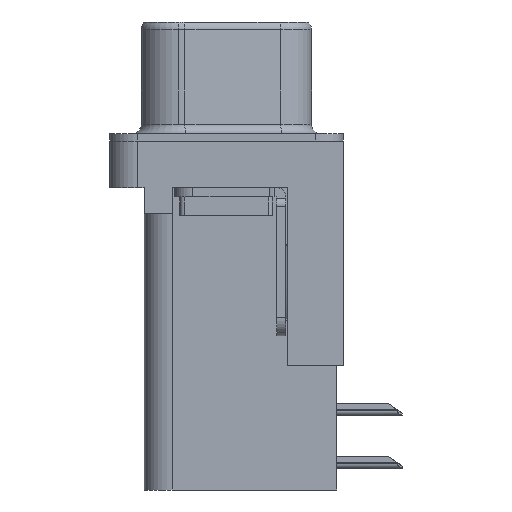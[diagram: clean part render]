
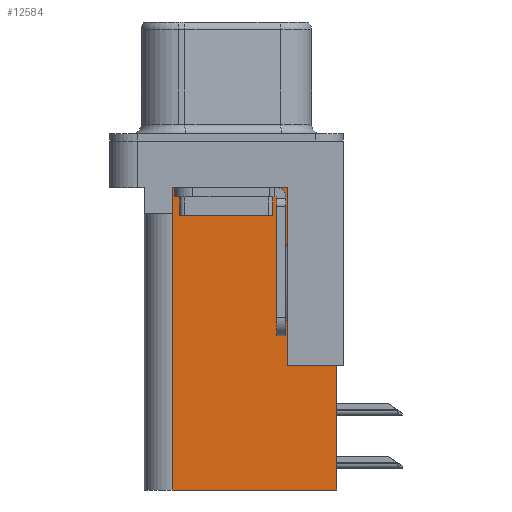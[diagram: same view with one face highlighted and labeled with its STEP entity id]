
A CAD part, left-side view. The second image highlights one B-rep face of the part: STEP entity #12584.
In plain terms, the highlighted planar face has unit normal (-1, 0, 0).
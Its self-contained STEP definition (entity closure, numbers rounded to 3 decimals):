
#171 = CARTESIAN_POINT ( 'NONE',  ( 3.7, -3.295, -18.76 ) ) ;
#661 = CARTESIAN_POINT ( 'NONE',  ( 3.7, 2.895, -3.9 ) ) ;
#1415 = CARTESIAN_POINT ( 'NONE',  ( 3.7, -3.295, -18.76 ) ) ;
#1554 = VECTOR ( 'NONE', #4974, 1000. ) ;
#1635 = LINE ( 'NONE', #19771, #1554 ) ;
#2069 = CARTESIAN_POINT ( 'NONE',  ( 3.7, -3.295, -2.5 ) ) ;
#3405 = VERTEX_POINT ( 'NONE', #21352 ) ;
#3714 = CARTESIAN_POINT ( 'NONE',  ( 3.7, 2.925, -18.76 ) ) ;
#3831 = CARTESIAN_POINT ( 'NONE',  ( 3.7, -6.295, -12.05 ) ) ;
#3982 = EDGE_LOOP ( 'NONE', ( #12504, #12738, #13119, #13442, #16560, #17139, #17426, #17558 ) ) ;
#4039 = VERTEX_POINT ( 'NONE', #17982 ) ;
#4243 = DIRECTION ( 'NONE',  ( 0., 1., 0. ) ) ;
#4322 = CARTESIAN_POINT ( 'NONE',  ( 3.7, 2.895, -3.9 ) ) ;
#4974 = DIRECTION ( 'NONE',  ( 0., 1., 0. ) ) ;
#6095 = DIRECTION ( 'NONE',  ( 0., 1., 0. ) ) ;
#6292 = DIRECTION ( 'NONE',  ( 0., 0., 1. ) ) ;
#6376 = VECTOR ( 'NONE', #6292, 1000. ) ;
#6480 = VERTEX_POINT ( 'NONE', #16243 ) ;
#6636 = LINE ( 'NONE', #171, #6376 ) ;
#6810 = CARTESIAN_POINT ( 'NONE',  ( 3.7, 2.925, -3.9 ) ) ;
#6896 = EDGE_CURVE ( 'NONE', #7898, #15439, #16103, .T. ) ;
#6897 = VECTOR ( 'NONE', #17127, 1000. ) ;
#6919 = LINE ( 'NONE', #3831, #6897 ) ;
#7898 = VERTEX_POINT ( 'NONE', #18029 ) ;
#8158 = LINE ( 'NONE', #13703, #8191 ) ;
#8191 = VECTOR ( 'NONE', #13785, 1000. ) ;
#8558 = VECTOR ( 'NONE', #12336, 1000. ) ;
#8704 = LINE ( 'NONE', #14214, #8558 ) ;
#8971 = EDGE_CURVE ( 'NONE', #4039, #7898, #8704, .T. ) ;
#9115 = EDGE_CURVE ( 'NONE', #13469, #4039, #8158, .T. ) ;
#9572 = EDGE_CURVE ( 'NONE', #13469, #16283, #6919, .T. ) ;
#9633 = DIRECTION ( 'NONE',  ( 0., 0., 1. ) ) ;
#9721 = EDGE_CURVE ( 'NONE', #16283, #3405, #6636, .T. ) ;
#11568 = VECTOR ( 'NONE', #19275, 1000. ) ;
#11760 = LINE ( 'NONE', #4322, #11568 ) ;
#12336 = DIRECTION ( 'NONE',  ( 0., 1., 0. ) ) ;
#12504 = ORIENTED_EDGE ( 'NONE', *, *, #18961, .T. ) ;
#12584 = ADVANCED_FACE ( 'NONE', ( #23570 ), #13771, .F. ) ;
#12738 = ORIENTED_EDGE ( 'NONE', *, *, #21416, .T. ) ;
#13119 = ORIENTED_EDGE ( 'NONE', *, *, #23737, .T. ) ;
#13442 = ORIENTED_EDGE ( 'NONE', *, *, #6896, .F. ) ;
#13469 = VERTEX_POINT ( 'NONE', #21233 ) ;
#13703 = CARTESIAN_POINT ( 'NONE',  ( 3.7, -5.925, -2. ) ) ;
#13771 = PLANE ( 'NONE',  #21087 ) ;
#13785 = DIRECTION ( 'NONE',  ( 0., 0., -1. ) ) ;
#14214 = CARTESIAN_POINT ( 'NONE',  ( 3.7, -3.295, -18.76 ) ) ;
#14871 = CARTESIAN_POINT ( 'NONE',  ( 3.7, -3.295, -12.05 ) ) ;
#15439 = VERTEX_POINT ( 'NONE', #6810 ) ;
#15578 = DIRECTION ( 'NONE',  ( 1., 0., 0. ) ) ;
#16079 = VECTOR ( 'NONE', #9633, 1000. ) ;
#16103 = LINE ( 'NONE', #3714, #16079 ) ;
#16243 = CARTESIAN_POINT ( 'NONE',  ( 3.7, 2.895, -2.5 ) ) ;
#16283 = VERTEX_POINT ( 'NONE', #14871 ) ;
#16560 = ORIENTED_EDGE ( 'NONE', *, *, #8971, .F. ) ;
#17127 = DIRECTION ( 'NONE',  ( 0., 1., 0. ) ) ;
#17139 = ORIENTED_EDGE ( 'NONE', *, *, #9115, .F. ) ;
#17338 = VECTOR ( 'NONE', #6095, 1000. ) ;
#17344 = LINE ( 'NONE', #2069, #17338 ) ;
#17426 = ORIENTED_EDGE ( 'NONE', *, *, #9572, .T. ) ;
#17558 = ORIENTED_EDGE ( 'NONE', *, *, #9721, .T. ) ;
#17982 = CARTESIAN_POINT ( 'NONE',  ( 3.7, -5.925, -18.76 ) ) ;
#18029 = CARTESIAN_POINT ( 'NONE',  ( 3.7, 2.925, -18.76 ) ) ;
#18961 = EDGE_CURVE ( 'NONE', #3405, #6480, #17344, .T. ) ;
#19275 = DIRECTION ( 'NONE',  ( 0., 0., -1. ) ) ;
#19771 = CARTESIAN_POINT ( 'NONE',  ( 3.7, 0., -3.9 ) ) ;
#20929 = VERTEX_POINT ( 'NONE', #661 ) ;
#21087 = AXIS2_PLACEMENT_3D ( 'NONE', #1415, #15578, #4243 ) ;
#21233 = CARTESIAN_POINT ( 'NONE',  ( 3.7, -5.925, -12.05 ) ) ;
#21352 = CARTESIAN_POINT ( 'NONE',  ( 3.7, -3.295, -2.5 ) ) ;
#21416 = EDGE_CURVE ( 'NONE', #6480, #20929, #11760, .T. ) ;
#23570 = FACE_OUTER_BOUND ( 'NONE', #3982, .T. ) ;
#23737 = EDGE_CURVE ( 'NONE', #20929, #15439, #1635, .T. ) ;
